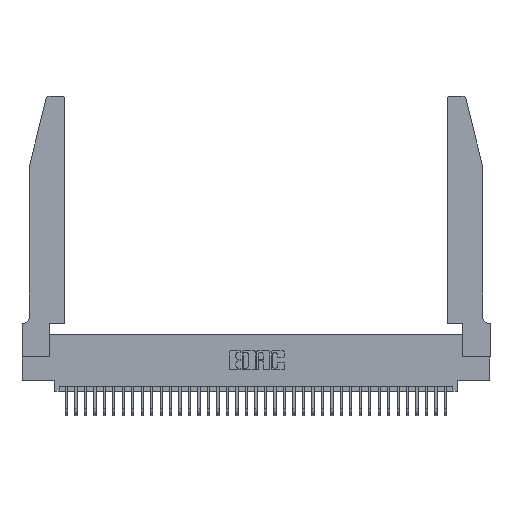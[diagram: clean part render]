
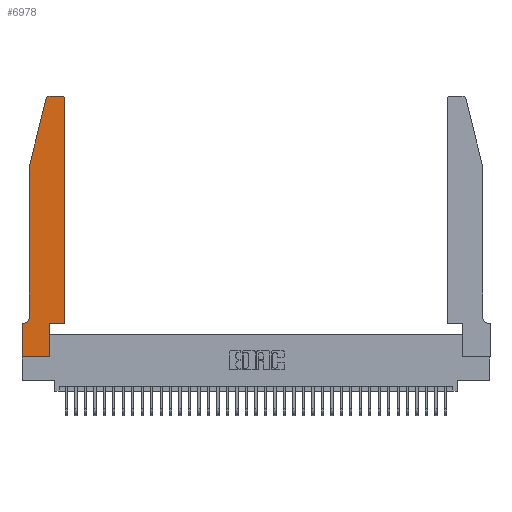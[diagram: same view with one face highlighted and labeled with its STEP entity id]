
A CAD part, top view. The second image highlights one B-rep face of the part: STEP entity #6978.
In plain terms, the highlighted planar face has unit normal (0, 0, 1).
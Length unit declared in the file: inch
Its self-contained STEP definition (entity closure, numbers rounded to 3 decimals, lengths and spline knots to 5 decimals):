
#113 = CARTESIAN_POINT ( 'NONE',  ( 0.2865, 0., 0.37 ) ) ;
#1107 = EDGE_CURVE ( 'NONE', #17797, #33331, #26705, .T. ) ;
#1776 = CARTESIAN_POINT ( 'NONE',  ( 0.4505, 0.35, 0.37 ) ) ;
#1949 = CARTESIAN_POINT ( 'NONE',  ( 0.0055, 0.42, 0.37 ) ) ;
#2971 = CARTESIAN_POINT ( 'NONE',  ( 0.0755, 2., 0.37 ) ) ;
#3222 = ORIENTED_EDGE ( 'NONE', *, *, #29745, .T. ) ;
#3535 = ORIENTED_EDGE ( 'NONE', *, *, #4487, .T. ) ;
#3812 = CARTESIAN_POINT ( 'NONE',  ( 0.2865, 0.35, 0.37 ) ) ;
#4365 = DIRECTION ( 'NONE',  ( 0., 0., 1. ) ) ;
#4487 = EDGE_CURVE ( 'NONE', #29779, #5156, #32835, .T. ) ;
#4514 = VECTOR ( 'NONE', #14258, 39.37008 ) ;
#4712 = DIRECTION ( 'NONE',  ( -1., 0., 0. ) ) ;
#5156 = VERTEX_POINT ( 'NONE', #30145 ) ;
#5332 = VERTEX_POINT ( 'NONE', #8614 ) ;
#5351 = VERTEX_POINT ( 'NONE', #33634 ) ;
#6200 = LINE ( 'NONE', #19049, #35787 ) ;
#6978 = ADVANCED_FACE ( 'NONE', ( #23477 ), #21953, .T. ) ;
#7759 = LINE ( 'NONE', #3812, #28176 ) ;
#8042 = CARTESIAN_POINT ( 'NONE',  ( 0.25487, 2.72718, 0.37 ) ) ;
#8106 = DIRECTION ( 'NONE',  ( 1., 0., 0. ) ) ;
#8513 = VERTEX_POINT ( 'NONE', #8042 ) ;
#8614 = CARTESIAN_POINT ( 'NONE',  ( 0.2865, 0.35, 0.37 ) ) ;
#8894 = EDGE_CURVE ( 'NONE', #33331, #29779, #19860, .T. ) ;
#8971 = CIRCLE ( 'NONE', #17455, 0.07 ) ;
#9496 = DIRECTION ( 'NONE',  ( -1., 0., 0. ) ) ;
#9856 = VERTEX_POINT ( 'NONE', #22913 ) ;
#10574 = EDGE_CURVE ( 'NONE', #9856, #20963, #8971, .T. ) ;
#10883 = AXIS2_PLACEMENT_3D ( 'NONE', #19161, #24745, #8106 ) ;
#11263 = ORIENTED_EDGE ( 'NONE', *, *, #11880, .T. ) ;
#11880 = EDGE_CURVE ( 'NONE', #8513, #18298, #25387, .T. ) ;
#11958 = DIRECTION ( 'NONE',  ( 0., 0., 1. ) ) ;
#13009 = ORIENTED_EDGE ( 'NONE', *, *, #1107, .T. ) ;
#13474 = DIRECTION ( 'NONE',  ( 1., 0., 0. ) ) ;
#14109 = EDGE_CURVE ( 'NONE', #23496, #5351, #25216, .T. ) ;
#14170 = CARTESIAN_POINT ( 'NONE',  ( 0.4205, 2.75, 0.37 ) ) ;
#14258 = DIRECTION ( 'NONE',  ( 0., 1., 0. ) ) ;
#15523 = DIRECTION ( 'NONE',  ( -0.239, -0.971, 0. ) ) ;
#15841 = LINE ( 'NONE', #2971, #23207 ) ;
#17196 = AXIS2_PLACEMENT_3D ( 'NONE', #21014, #4365, #23818 ) ;
#17455 = AXIS2_PLACEMENT_3D ( 'NONE', #1949, #21366, #4712 ) ;
#17651 = ORIENTED_EDGE ( 'NONE', *, *, #30789, .T. ) ;
#17660 = EDGE_CURVE ( 'NONE', #31780, #5332, #7759, .T. ) ;
#17797 = VERTEX_POINT ( 'NONE', #1776 ) ;
#17821 = VECTOR ( 'NONE', #28298, 39.37008 ) ;
#17995 = VECTOR ( 'NONE', #15523, 39.37008 ) ;
#18044 = VECTOR ( 'NONE', #35015, 39.37008 ) ;
#18298 = VERTEX_POINT ( 'NONE', #23099 ) ;
#18416 = LINE ( 'NONE', #26139, #25799 ) ;
#18647 = AXIS2_PLACEMENT_3D ( 'NONE', #28580, #11958, #31370 ) ;
#18984 = ORIENTED_EDGE ( 'NONE', *, *, #23252, .T. ) ;
#19024 = ORIENTED_EDGE ( 'NONE', *, *, #14109, .T. ) ;
#19049 = CARTESIAN_POINT ( 'NONE',  ( 0., 0., 0.37 ) ) ;
#19161 = CARTESIAN_POINT ( 'NONE',  ( 0., 0.35, 0.37 ) ) ;
#19604 = DIRECTION ( 'NONE',  ( 0., -1., 0. ) ) ;
#19685 = CARTESIAN_POINT ( 'NONE',  ( 0.4505, 0.35, 0.37 ) ) ;
#19860 = CIRCLE ( 'NONE', #17196, 0.03 ) ;
#20111 = CARTESIAN_POINT ( 'NONE',  ( 0.0055, 0.35, 0.37 ) ) ;
#20184 = EDGE_CURVE ( 'NONE', #5332, #17797, #33207, .T. ) ;
#20453 = DIRECTION ( 'NONE',  ( 0., 1., 0. ) ) ;
#20963 = VERTEX_POINT ( 'NONE', #20111 ) ;
#21014 = CARTESIAN_POINT ( 'NONE',  ( 0.4205, 2.72, 0.37 ) ) ;
#21366 = DIRECTION ( 'NONE',  ( 0., 0., -1. ) ) ;
#21953 = PLANE ( 'NONE',  #10883 ) ;
#22478 = DIRECTION ( 'NONE',  ( 1., 0., 0. ) ) ;
#22720 = CARTESIAN_POINT ( 'NONE',  ( 0., 0., 0.37 ) ) ;
#22913 = CARTESIAN_POINT ( 'NONE',  ( 0.0755, 0.42, 0.37 ) ) ;
#23099 = CARTESIAN_POINT ( 'NONE',  ( 0.0755, 2., 0.37 ) ) ;
#23207 = VECTOR ( 'NONE', #19604, 39.37008 ) ;
#23252 = EDGE_CURVE ( 'NONE', #5351, #31780, #6200, .T. ) ;
#23477 = FACE_OUTER_BOUND ( 'NONE', #33251, .T. ) ;
#23496 = VERTEX_POINT ( 'NONE', #28373 ) ;
#23818 = DIRECTION ( 'NONE',  ( 1., 0., 0. ) ) ;
#24582 = EDGE_CURVE ( 'NONE', #5156, #8513, #28764, .T. ) ;
#24745 = DIRECTION ( 'NONE',  ( 0., 0., 1. ) ) ;
#25216 = LINE ( 'NONE', #22720, #17821 ) ;
#25317 = ORIENTED_EDGE ( 'NONE', *, *, #20184, .T. ) ;
#25387 = LINE ( 'NONE', #26569, #17995 ) ;
#25799 = VECTOR ( 'NONE', #9496, 39.37008 ) ;
#26069 = ORIENTED_EDGE ( 'NONE', *, *, #17660, .T. ) ;
#26139 = CARTESIAN_POINT ( 'NONE',  ( 0.0755, 0.35, 0.37 ) ) ;
#26569 = CARTESIAN_POINT ( 'NONE',  ( 0.0755, 2., 0.37 ) ) ;
#26694 = VECTOR ( 'NONE', #22478, 39.37008 ) ;
#26705 = LINE ( 'NONE', #28079, #4514 ) ;
#26771 = CARTESIAN_POINT ( 'NONE',  ( 0.2605, 2.75, 0.37 ) ) ;
#27922 = ORIENTED_EDGE ( 'NONE', *, *, #24582, .T. ) ;
#28079 = CARTESIAN_POINT ( 'NONE',  ( 0.4505, 0.35, 0.37 ) ) ;
#28176 = VECTOR ( 'NONE', #20453, 39.37008 ) ;
#28298 = DIRECTION ( 'NONE',  ( 0., -1., 0. ) ) ;
#28373 = CARTESIAN_POINT ( 'NONE',  ( 0., 0.35, 0.37 ) ) ;
#28580 = CARTESIAN_POINT ( 'NONE',  ( 0.284, 2.72, 0.37 ) ) ;
#28764 = CIRCLE ( 'NONE', #18647, 0.03 ) ;
#29745 = EDGE_CURVE ( 'NONE', #18298, #9856, #15841, .T. ) ;
#29779 = VERTEX_POINT ( 'NONE', #14170 ) ;
#29966 = CARTESIAN_POINT ( 'NONE',  ( 0.4505, 2.72, 0.37 ) ) ;
#30145 = CARTESIAN_POINT ( 'NONE',  ( 0.284, 2.75, 0.37 ) ) ;
#30789 = EDGE_CURVE ( 'NONE', #20963, #23496, #18416, .T. ) ;
#31370 = DIRECTION ( 'NONE',  ( 1., 0., 0. ) ) ;
#31780 = VERTEX_POINT ( 'NONE', #113 ) ;
#32835 = LINE ( 'NONE', #26771, #18044 ) ;
#32970 = ORIENTED_EDGE ( 'NONE', *, *, #8894, .T. ) ;
#33207 = LINE ( 'NONE', #19685, #26694 ) ;
#33251 = EDGE_LOOP ( 'NONE', ( #3535, #27922, #11263, #3222, #35593, #17651, #19024, #18984, #26069, #25317, #13009, #32970 ) ) ;
#33331 = VERTEX_POINT ( 'NONE', #29966 ) ;
#33634 = CARTESIAN_POINT ( 'NONE',  ( 0., 0., 0.37 ) ) ;
#35015 = DIRECTION ( 'NONE',  ( -1., 0., 0. ) ) ;
#35593 = ORIENTED_EDGE ( 'NONE', *, *, #10574, .T. ) ;
#35787 = VECTOR ( 'NONE', #13474, 39.37008 ) ;
